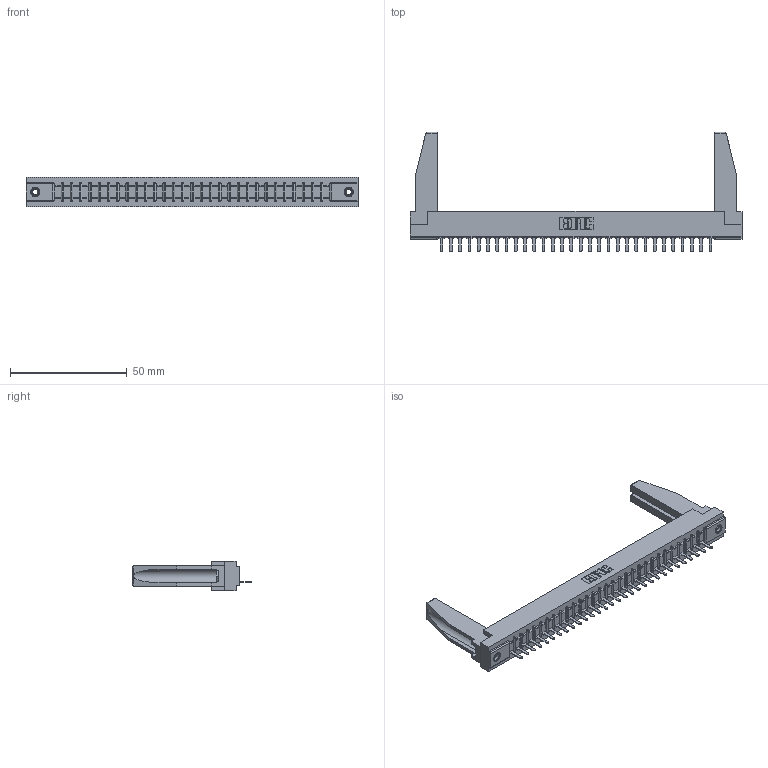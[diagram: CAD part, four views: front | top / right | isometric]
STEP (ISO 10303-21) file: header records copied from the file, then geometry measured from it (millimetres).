
FILE_DESCRIPTION (( 'STEP AP203' ), '1' );
FILE_NAME ('357-030-421-178.STEP', '2020-10-02T01:38:10', ( '' ), ( '' ), 'SwSTEP 2.0', 'SolidWorks 2020', '' );
FILE_SCHEMA (( 'CONFIG_CONTROL_DESIGN' ));
Length unit declared in the file: inch
Products named in the file (5): 307-220-078; 345-250-001_345-250-001-102; 357-030-421-178; 307 Part_.156 Dia Mounting Holes; 307-290-002_521
Assembly tree (35 placements, depth 2):
  357-030-421-178
    307 Part_.156 Dia Mounting Holes
    307-290-002_521  x30
    307-220-078  x2
    345-250-001_345-250-001-102  x2
Bounding box: 141.88 x 51.13 x 12.7 mm (x, y, z)
Volume: 19089 mm3; surface area: 22548.4 mm2
Topology: 35 solids, 35 shells, 2499 faces, 7613 edges, 4982 vertices
Faces by surface type: plane 1504, cylinder 917, sphere 62, cone 12, torus 4
Entity records: 30355 total; most frequent: CARTESIAN_POINT 5118, ORIENTED_EDGE 5064, DIRECTION 4934, EDGE_CURVE 2532, VECTOR 1938, LINE 1938, VERTEX_POINT 1640, AXIS2_PLACEMENT_3D 1498
